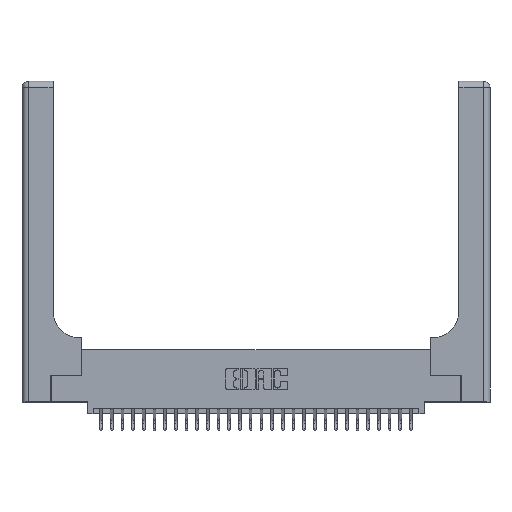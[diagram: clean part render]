
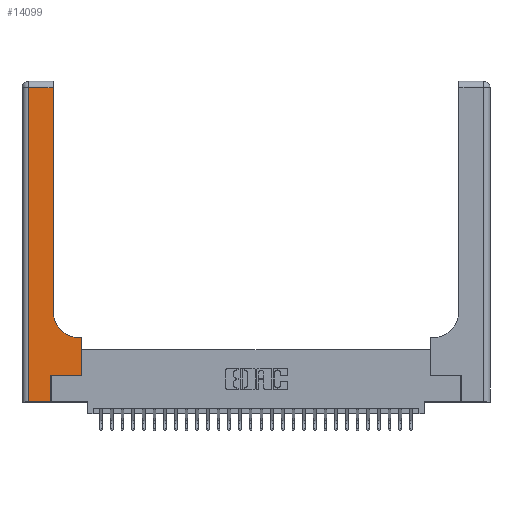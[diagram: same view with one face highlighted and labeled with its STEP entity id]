
A CAD part, top view. The second image highlights one B-rep face of the part: STEP entity #14099.
In plain terms, the highlighted planar face has unit normal (0, 0, 1).
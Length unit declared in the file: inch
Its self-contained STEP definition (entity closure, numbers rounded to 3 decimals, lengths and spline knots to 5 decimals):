
#39 = LINE ( 'NONE', #25909, #23855 ) ;
#58 = CARTESIAN_POINT ( 'NONE',  ( 0.06, 0., 0.37 ) ) ;
#113 = VECTOR ( 'NONE', #16463, 39.37008 ) ;
#1558 = VECTOR ( 'NONE', #6665, 39.37008 ) ;
#1596 = VERTEX_POINT ( 'NONE', #23130 ) ;
#1624 = DIRECTION ( 'NONE',  ( -1., 0., 0. ) ) ;
#1738 = VECTOR ( 'NONE', #28482, 39.37008 ) ;
#2028 = DIRECTION ( 'NONE',  ( 1., 0., 0. ) ) ;
#2813 = CARTESIAN_POINT ( 'NONE',  ( 0.5585, 0.25, 0.37 ) ) ;
#3029 = CARTESIAN_POINT ( 'NONE',  ( 0.2915, 2.94, 0.37 ) ) ;
#3333 = DIRECTION ( 'NONE',  ( 1., 0., 0. ) ) ;
#4281 = ORIENTED_EDGE ( 'NONE', *, *, #22643, .T. ) ;
#4354 = CARTESIAN_POINT ( 'NONE',  ( 0., 3., 0.37 ) ) ;
#4642 = CARTESIAN_POINT ( 'NONE',  ( 0.06, 3., 0.37 ) ) ;
#5256 = EDGE_CURVE ( 'NONE', #12266, #30336, #18327, .T. ) ;
#6539 = VERTEX_POINT ( 'NONE', #16610 ) ;
#6650 = EDGE_CURVE ( 'NONE', #18668, #1596, #18240, .T. ) ;
#6661 = CARTESIAN_POINT ( 'NONE',  ( 0.06, 2.94, 0.37 ) ) ;
#6665 = DIRECTION ( 'NONE',  ( 1., 0., 0. ) ) ;
#7474 = DIRECTION ( 'NONE',  ( 0., 1., 0. ) ) ;
#8276 = LINE ( 'NONE', #12142, #13850 ) ;
#8601 = VECTOR ( 'NONE', #3333, 39.37008 ) ;
#8695 = ORIENTED_EDGE ( 'NONE', *, *, #30204, .T. ) ;
#8963 = FACE_OUTER_BOUND ( 'NONE', #24232, .T. ) ;
#9005 = EDGE_CURVE ( 'NONE', #6539, #11953, #17337, .T. ) ;
#9995 = VERTEX_POINT ( 'NONE', #27708 ) ;
#10311 = CARTESIAN_POINT ( 'NONE',  ( 0.2915, 0.85, 0.37 ) ) ;
#11898 = CARTESIAN_POINT ( 'NONE',  ( 0.269, 0., 0.37 ) ) ;
#11953 = VERTEX_POINT ( 'NONE', #10311 ) ;
#12142 = CARTESIAN_POINT ( 'NONE',  ( 0.269, 0., 0.37 ) ) ;
#12266 = VERTEX_POINT ( 'NONE', #6661 ) ;
#12490 = EDGE_CURVE ( 'NONE', #24492, #9995, #8276, .T. ) ;
#13835 = EDGE_CURVE ( 'NONE', #9995, #18668, #14928, .T. ) ;
#13850 = VECTOR ( 'NONE', #7474, 39.37008 ) ;
#13875 = DIRECTION ( 'NONE',  ( -1., 0., 0. ) ) ;
#13979 = DIRECTION ( 'NONE',  ( 0., 1., 0. ) ) ;
#14099 = ADVANCED_FACE ( 'NONE', ( #8963 ), #18609, .F. ) ;
#14325 = LINE ( 'NONE', #26140, #1738 ) ;
#14928 = LINE ( 'NONE', #24785, #8601 ) ;
#15585 = ORIENTED_EDGE ( 'NONE', *, *, #18946, .T. ) ;
#15954 = ORIENTED_EDGE ( 'NONE', *, *, #13835, .T. ) ;
#16241 = DIRECTION ( 'NONE',  ( 0., 0., -1. ) ) ;
#16463 = DIRECTION ( 'NONE',  ( 0., -1., 0. ) ) ;
#16610 = CARTESIAN_POINT ( 'NONE',  ( 0.5415, 0.6, 0.37 ) ) ;
#17337 = CIRCLE ( 'NONE', #23734, 0.25 ) ;
#17558 = LINE ( 'NONE', #30053, #23173 ) ;
#18016 = AXIS2_PLACEMENT_3D ( 'NONE', #4354, #28134, #13875 ) ;
#18240 = LINE ( 'NONE', #2813, #24576 ) ;
#18327 = LINE ( 'NONE', #4642, #113 ) ;
#18507 = ORIENTED_EDGE ( 'NONE', *, *, #12490, .T. ) ;
#18550 = CARTESIAN_POINT ( 'NONE',  ( 0., 0., 0.37 ) ) ;
#18609 = PLANE ( 'NONE',  #18016 ) ;
#18668 = VERTEX_POINT ( 'NONE', #27179 ) ;
#18946 = EDGE_CURVE ( 'NONE', #1596, #6539, #14325, .T. ) ;
#19469 = DIRECTION ( 'NONE',  ( 0., 1., 0. ) ) ;
#20518 = LINE ( 'NONE', #18550, #1558 ) ;
#20888 = VERTEX_POINT ( 'NONE', #3029 ) ;
#21800 = ORIENTED_EDGE ( 'NONE', *, *, #24425, .T. ) ;
#22643 = EDGE_CURVE ( 'NONE', #20888, #12266, #17558, .T. ) ;
#23130 = CARTESIAN_POINT ( 'NONE',  ( 0.5585, 0.6, 0.37 ) ) ;
#23173 = VECTOR ( 'NONE', #1624, 39.37008 ) ;
#23488 = ORIENTED_EDGE ( 'NONE', *, *, #9005, .T. ) ;
#23734 = AXIS2_PLACEMENT_3D ( 'NONE', #30457, #16241, #2028 ) ;
#23855 = VECTOR ( 'NONE', #13979, 39.37008 ) ;
#24232 = EDGE_LOOP ( 'NONE', ( #21800, #4281, #26126, #8695, #18507, #15954, #26813, #15585, #23488 ) ) ;
#24425 = EDGE_CURVE ( 'NONE', #11953, #20888, #39, .T. ) ;
#24492 = VERTEX_POINT ( 'NONE', #11898 ) ;
#24576 = VECTOR ( 'NONE', #19469, 39.37008 ) ;
#24785 = CARTESIAN_POINT ( 'NONE',  ( 0.269, 0.25, 0.37 ) ) ;
#25909 = CARTESIAN_POINT ( 'NONE',  ( 0.2915, 3., 0.37 ) ) ;
#26126 = ORIENTED_EDGE ( 'NONE', *, *, #5256, .T. ) ;
#26140 = CARTESIAN_POINT ( 'NONE',  ( 0.2915, 0.6, 0.37 ) ) ;
#26813 = ORIENTED_EDGE ( 'NONE', *, *, #6650, .T. ) ;
#27179 = CARTESIAN_POINT ( 'NONE',  ( 0.5585, 0.25, 0.37 ) ) ;
#27708 = CARTESIAN_POINT ( 'NONE',  ( 0.269, 0.25, 0.37 ) ) ;
#28134 = DIRECTION ( 'NONE',  ( 0., 0., -1. ) ) ;
#28482 = DIRECTION ( 'NONE',  ( -1., 0., 0. ) ) ;
#30053 = CARTESIAN_POINT ( 'NONE',  ( 0., 2.94, 0.37 ) ) ;
#30204 = EDGE_CURVE ( 'NONE', #30336, #24492, #20518, .T. ) ;
#30336 = VERTEX_POINT ( 'NONE', #58 ) ;
#30457 = CARTESIAN_POINT ( 'NONE',  ( 0.5415, 0.85, 0.37 ) ) ;
